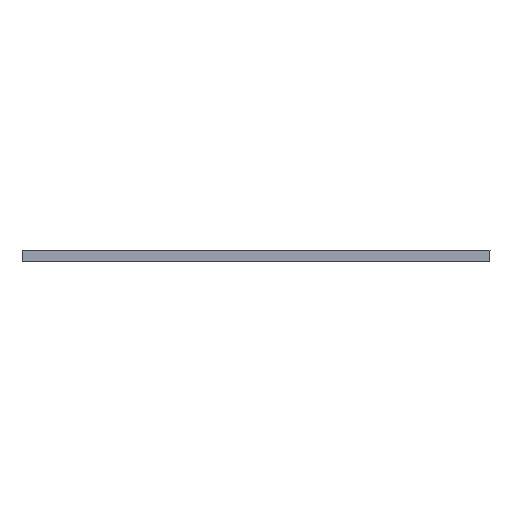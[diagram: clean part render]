
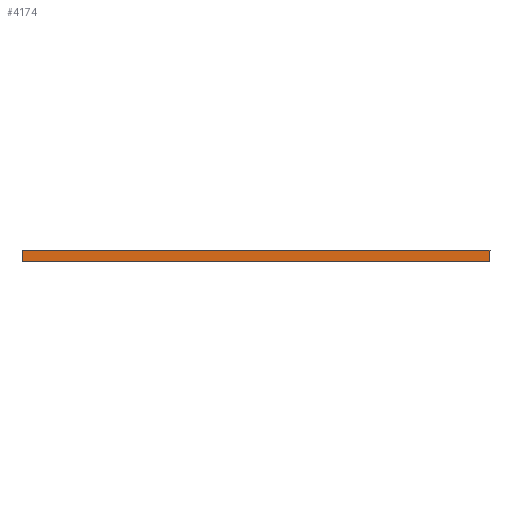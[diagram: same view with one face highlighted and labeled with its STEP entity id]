
A CAD part, left-side view. The second image highlights one B-rep face of the part: STEP entity #4174.
In plain terms, the highlighted planar face has unit normal (-1, 0, 0).
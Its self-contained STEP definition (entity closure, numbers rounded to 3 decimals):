
#99 = VERTEX_POINT ( 'NONE', #6603 ) ;
#141 = LINE ( 'NONE', #3933, #6633 ) ;
#344 = LINE ( 'NONE', #4298, #1759 ) ;
#347 = AXIS2_PLACEMENT_3D ( 'NONE', #6436, #7480, #4285 ) ;
#408 = VERTEX_POINT ( 'NONE', #1079 ) ;
#614 = LINE ( 'NONE', #5329, #5628 ) ;
#843 = ORIENTED_EDGE ( 'NONE', *, *, #1472, .F. ) ;
#1079 = CARTESIAN_POINT ( 'NONE',  ( -22.811, 20.5, 22.127 ) ) ;
#1311 = FACE_OUTER_BOUND ( 'NONE', #5810, .T. ) ;
#1434 = ORIENTED_EDGE ( 'NONE', *, *, #2145, .F. ) ;
#1472 = EDGE_CURVE ( 'NONE', #408, #99, #614, .T. ) ;
#1759 = VECTOR ( 'NONE', #4309, 1000. ) ;
#2128 = EDGE_CURVE ( 'NONE', #408, #3746, #141, .T. ) ;
#2141 = EDGE_CURVE ( 'NONE', #3746, #6704, #344, .T. ) ;
#2145 = EDGE_CURVE ( 'NONE', #99, #6704, #5102, .T. ) ;
#2250 = CARTESIAN_POINT ( 'NONE',  ( -22.811, -19.5, 21.127 ) ) ;
#2515 = ORIENTED_EDGE ( 'NONE', *, *, #2128, .T. ) ;
#2880 = DIRECTION ( 'NONE',  ( 0., 0., -1. ) ) ;
#2888 = CARTESIAN_POINT ( 'NONE',  ( -22.811, -19.5, 22.127 ) ) ;
#3619 = PLANE ( 'NONE',  #347 ) ;
#3746 = VERTEX_POINT ( 'NONE', #4731 ) ;
#3807 = DIRECTION ( 'NONE',  ( 0., 0., -1. ) ) ;
#3933 = CARTESIAN_POINT ( 'NONE',  ( -22.811, 20.5, 22.127 ) ) ;
#4174 = ADVANCED_FACE ( 'NONE', ( #1311 ), #3619, .F. ) ;
#4285 = DIRECTION ( 'NONE',  ( 0., 1., 0. ) ) ;
#4298 = CARTESIAN_POINT ( 'NONE',  ( -22.811, 20.5, 21.127 ) ) ;
#4309 = DIRECTION ( 'NONE',  ( 0., -1., 0. ) ) ;
#4731 = CARTESIAN_POINT ( 'NONE',  ( -22.811, 20.5, 21.127 ) ) ;
#5102 = LINE ( 'NONE', #2888, #5245 ) ;
#5245 = VECTOR ( 'NONE', #2880, 1000. ) ;
#5329 = CARTESIAN_POINT ( 'NONE',  ( -22.811, 20.5, 22.127 ) ) ;
#5606 = DIRECTION ( 'NONE',  ( 0., -1., 0. ) ) ;
#5628 = VECTOR ( 'NONE', #5606, 1000. ) ;
#5810 = EDGE_LOOP ( 'NONE', ( #6358, #1434, #843, #2515 ) ) ;
#6358 = ORIENTED_EDGE ( 'NONE', *, *, #2141, .T. ) ;
#6436 = CARTESIAN_POINT ( 'NONE',  ( -22.811, 20.5, 22.127 ) ) ;
#6603 = CARTESIAN_POINT ( 'NONE',  ( -22.811, -19.5, 22.127 ) ) ;
#6633 = VECTOR ( 'NONE', #3807, 1000. ) ;
#6704 = VERTEX_POINT ( 'NONE', #2250 ) ;
#7480 = DIRECTION ( 'NONE',  ( 1., 0., 0. ) ) ;
